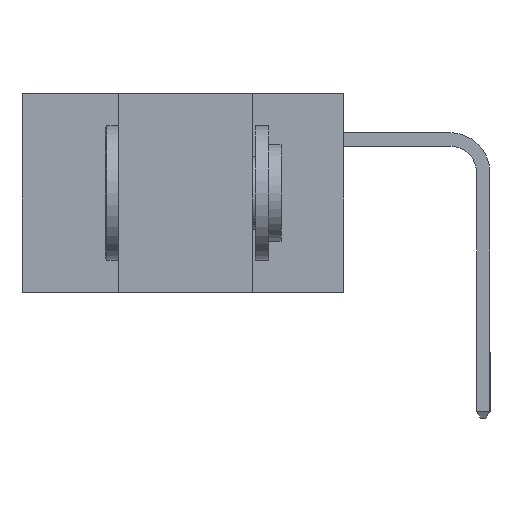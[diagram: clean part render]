
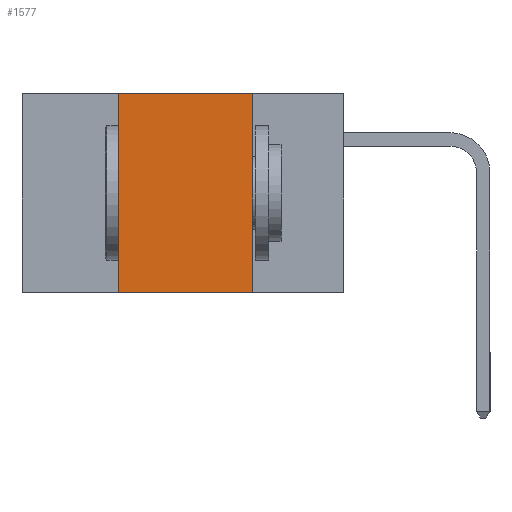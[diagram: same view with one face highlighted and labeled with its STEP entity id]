
A CAD part, left-side view. The second image highlights one B-rep face of the part: STEP entity #1577.
In plain terms, the highlighted planar face has unit normal (-1, 0, 0).
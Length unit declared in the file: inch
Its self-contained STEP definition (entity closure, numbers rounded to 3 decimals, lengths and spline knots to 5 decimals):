
#13 = CARTESIAN_POINT ( 'NONE',  ( 0., 0.42, -0.37 ) ) ;
#336 = PLANE ( 'NONE',  #9940 ) ;
#748 = DIRECTION ( 'NONE',  ( 0., -1., 0. ) ) ;
#1531 = DIRECTION ( 'NONE',  ( 0., -1., 0. ) ) ;
#1577 = ADVANCED_FACE ( 'NONE', ( #10143 ), #336, .F. ) ;
#1867 = VERTEX_POINT ( 'NONE', #10710 ) ;
#2598 = DIRECTION ( 'NONE',  ( 0., 0., -1. ) ) ;
#2704 = EDGE_CURVE ( 'NONE', #8414, #1867, #7469, .T. ) ;
#3391 = VECTOR ( 'NONE', #748, 39.37008 ) ;
#3578 = CARTESIAN_POINT ( 'NONE',  ( 0., 0.42, 0. ) ) ;
#3623 = VECTOR ( 'NONE', #9781, 39.37008 ) ;
#3760 = VECTOR ( 'NONE', #2598, 39.37008 ) ;
#3961 = VERTEX_POINT ( 'NONE', #7600 ) ;
#4214 = LINE ( 'NONE', #11467, #3760 ) ;
#4245 = LINE ( 'NONE', #7039, #3623 ) ;
#4357 = CARTESIAN_POINT ( 'NONE',  ( 0., 0.6, 0. ) ) ;
#4393 = EDGE_CURVE ( 'NONE', #10920, #3961, #7947, .T. ) ;
#4464 = ORIENTED_EDGE ( 'NONE', *, *, #2704, .T. ) ;
#6296 = CARTESIAN_POINT ( 'NONE',  ( 0., 0.6, -0.37 ) ) ;
#6752 = CARTESIAN_POINT ( 'NONE',  ( 0., 0.6, 0. ) ) ;
#6834 = DIRECTION ( 'NONE',  ( 1., 0., 0. ) ) ;
#7039 = CARTESIAN_POINT ( 'NONE',  ( 0., 0.42, 0. ) ) ;
#7469 = LINE ( 'NONE', #6296, #3391 ) ;
#7600 = CARTESIAN_POINT ( 'NONE',  ( 0., 0.17, 0. ) ) ;
#7947 = LINE ( 'NONE', #4357, #11588 ) ;
#8128 = ORIENTED_EDGE ( 'NONE', *, *, #4393, .F. ) ;
#8249 = EDGE_LOOP ( 'NONE', ( #11836, #8128, #9982, #4464 ) ) ;
#8293 = DIRECTION ( 'NONE',  ( 0., 0., -1. ) ) ;
#8414 = VERTEX_POINT ( 'NONE', #13 ) ;
#9781 = DIRECTION ( 'NONE',  ( 0., 0., 1. ) ) ;
#9823 = EDGE_CURVE ( 'NONE', #8414, #10920, #4245, .T. ) ;
#9940 = AXIS2_PLACEMENT_3D ( 'NONE', #6752, #6834, #8293 ) ;
#9982 = ORIENTED_EDGE ( 'NONE', *, *, #9823, .F. ) ;
#10143 = FACE_OUTER_BOUND ( 'NONE', #8249, .T. ) ;
#10710 = CARTESIAN_POINT ( 'NONE',  ( 0., 0.17, -0.37 ) ) ;
#10920 = VERTEX_POINT ( 'NONE', #3578 ) ;
#11467 = CARTESIAN_POINT ( 'NONE',  ( 0., 0.17, 0. ) ) ;
#11577 = EDGE_CURVE ( 'NONE', #3961, #1867, #4214, .T. ) ;
#11588 = VECTOR ( 'NONE', #1531, 39.37008 ) ;
#11836 = ORIENTED_EDGE ( 'NONE', *, *, #11577, .F. ) ;
